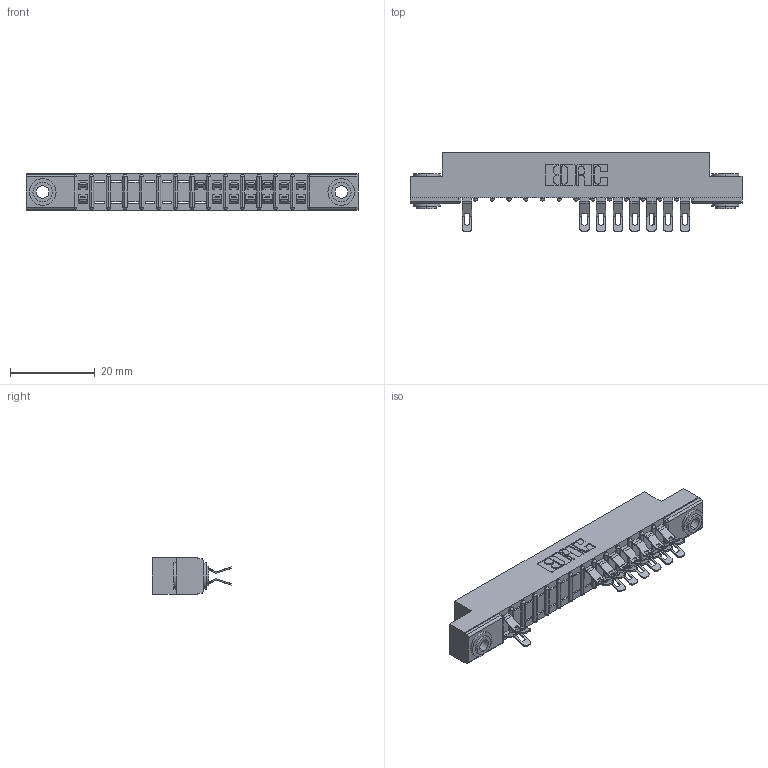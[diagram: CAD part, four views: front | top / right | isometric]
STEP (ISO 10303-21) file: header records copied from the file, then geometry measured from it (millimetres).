
FILE_DESCRIPTION (( 'STEP AP203' ), '1' );
FILE_NAME ('307-028-555-203.STEP', '2018-08-04T17:00:07', ( '' ), ( '' ), 'SwSTEP 2.0', 'SolidWorks 2016', '' );
FILE_SCHEMA (( 'CONFIG_CONTROL_DESIGN' ));
Length unit declared in the file: inch
Products named in the file (4): 307-290-001_555; 345-250-002_345-250-002-102; 307-028-555-203; 307 Part_.156 Dia Mounting Holes
Assembly tree (18 placements, depth 2):
  307-028-555-203
    307 Part_.156 Dia Mounting Holes
    307-290-001_555  x15
    345-250-002_345-250-002-102  x2
Bounding box: 78.49 x 18.75 x 8.71 mm (x, y, z)
Volume: 5012.4 mm3; surface area: 7936.1 mm2
Topology: 18 solids, 18 shells, 1230 faces, 3566 edges, 2312 vertices
Faces by surface type: plane 682, cylinder 510, sphere 30, cone 8
Entity records: 17088 total; most frequent: CARTESIAN_POINT 2846, ORIENTED_EDGE 2824, DIRECTION 2808, EDGE_CURVE 1412, LINE 1052, VECTOR 1052, VERTEX_POINT 916, AXIS2_PLACEMENT_3D 878
